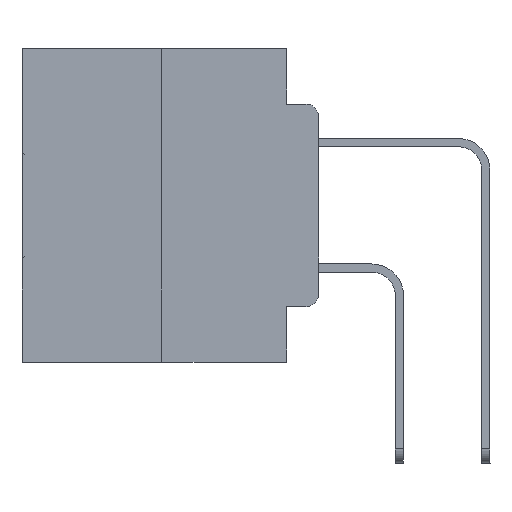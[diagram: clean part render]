
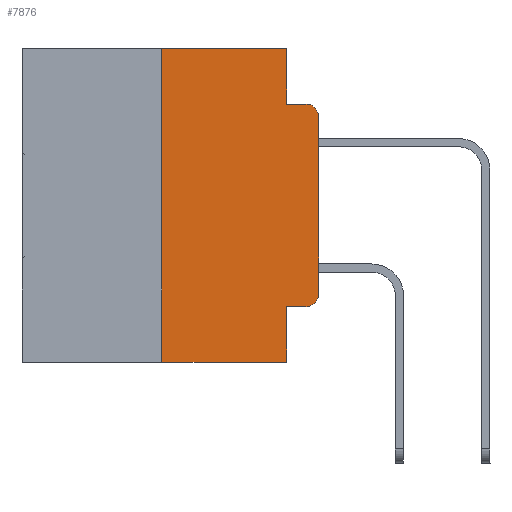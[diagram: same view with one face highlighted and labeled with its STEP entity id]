
A CAD part, left-side view. The second image highlights one B-rep face of the part: STEP entity #7876.
In plain terms, the highlighted planar face has unit normal (-1, 0, 0).
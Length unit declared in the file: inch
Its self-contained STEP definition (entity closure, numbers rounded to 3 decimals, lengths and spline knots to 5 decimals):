
#270 = VERTEX_POINT ( 'NONE', #4595 ) ;
#1238 = CARTESIAN_POINT ( 'NONE',  ( 0., 0.02, -0.3915 ) ) ;
#1372 = EDGE_CURVE ( 'NONE', #30174, #270, #13356, .T. ) ;
#1928 = VERTEX_POINT ( 'NONE', #25315 ) ;
#2842 = CARTESIAN_POINT ( 'NONE',  ( 0., 0.473, 0. ) ) ;
#2890 = VERTEX_POINT ( 'NONE', #15559 ) ;
#2945 = PLANE ( 'NONE',  #19170 ) ;
#3077 = EDGE_CURVE ( 'NONE', #2890, #270, #5493, .T. ) ;
#3279 = DIRECTION ( 'NONE',  ( 0., 0., 1. ) ) ;
#3811 = DIRECTION ( 'NONE',  ( 0., 0., -1. ) ) ;
#4303 = DIRECTION ( 'NONE',  ( 0., 0., -1. ) ) ;
#4576 = ORIENTED_EDGE ( 'NONE', *, *, #26491, .F. ) ;
#4595 = CARTESIAN_POINT ( 'NONE',  ( 0., 0.02, -0.0885 ) ) ;
#4787 = EDGE_CURVE ( 'NONE', #20805, #2890, #20725, .T. ) ;
#4844 = EDGE_LOOP ( 'NONE', ( #20172, #8056, #9629, #22399, #29525, #4576, #11192, #5338, #24660, #26188 ) ) ;
#4935 = VECTOR ( 'NONE', #18849, 39.37008 ) ;
#5258 = VECTOR ( 'NONE', #24513, 39.37008 ) ;
#5312 = LINE ( 'NONE', #20573, #29499 ) ;
#5338 = ORIENTED_EDGE ( 'NONE', *, *, #21654, .F. ) ;
#5465 = DIRECTION ( 'NONE',  ( 1., 0., 0. ) ) ;
#5493 = CIRCLE ( 'NONE', #10427, 0.02 ) ;
#5807 = CARTESIAN_POINT ( 'NONE',  ( 0., 0., 0. ) ) ;
#6363 = LINE ( 'NONE', #30226, #18552 ) ;
#6701 = CARTESIAN_POINT ( 'NONE',  ( 0., 0.25, -0.5 ) ) ;
#6771 = VECTOR ( 'NONE', #21631, 39.37008 ) ;
#6931 = DIRECTION ( 'NONE',  ( -1., 0., 0. ) ) ;
#7005 = CARTESIAN_POINT ( 'NONE',  ( 0., 0.02, -0.1085 ) ) ;
#7876 = ADVANCED_FACE ( 'NONE', ( #16884 ), #2945, .F. ) ;
#8056 = ORIENTED_EDGE ( 'NONE', *, *, #3077, .T. ) ;
#9015 = LINE ( 'NONE', #31048, #14792 ) ;
#9629 = ORIENTED_EDGE ( 'NONE', *, *, #1372, .F. ) ;
#10427 = AXIS2_PLACEMENT_3D ( 'NONE', #7005, #6931, #4303 ) ;
#11192 = ORIENTED_EDGE ( 'NONE', *, *, #26910, .T. ) ;
#11293 = CARTESIAN_POINT ( 'NONE',  ( 0., 0.051, -0.0885 ) ) ;
#11627 = CARTESIAN_POINT ( 'NONE',  ( 0., 0.25, 0. ) ) ;
#11630 = VERTEX_POINT ( 'NONE', #6701 ) ;
#12030 = CARTESIAN_POINT ( 'NONE',  ( 0., 0.051, 0. ) ) ;
#12297 = EDGE_CURVE ( 'NONE', #1928, #14678, #9015, .T. ) ;
#12622 = CARTESIAN_POINT ( 'NONE',  ( 0., 0.051, 0. ) ) ;
#13356 = LINE ( 'NONE', #11293, #6771 ) ;
#14461 = DIRECTION ( 'NONE',  ( 0., -1., 0. ) ) ;
#14678 = VERTEX_POINT ( 'NONE', #12030 ) ;
#14792 = VECTOR ( 'NONE', #14461, 39.37008 ) ;
#15109 = VERTEX_POINT ( 'NONE', #23163 ) ;
#15559 = CARTESIAN_POINT ( 'NONE',  ( 0., 0., -0.1085 ) ) ;
#16431 = LINE ( 'NONE', #17887, #28388 ) ;
#16884 = FACE_OUTER_BOUND ( 'NONE', #4844, .T. ) ;
#17194 = VERTEX_POINT ( 'NONE', #22791 ) ;
#17519 = LINE ( 'NONE', #12622, #5258 ) ;
#17887 = CARTESIAN_POINT ( 'NONE',  ( 0., 0.473, -0.5 ) ) ;
#17980 = AXIS2_PLACEMENT_3D ( 'NONE', #1238, #18458, #3811 ) ;
#18277 = DIRECTION ( 'NONE',  ( 0., -1., 0. ) ) ;
#18353 = DIRECTION ( 'NONE',  ( 0., 0., -1. ) ) ;
#18458 = DIRECTION ( 'NONE',  ( -1., 0., 0. ) ) ;
#18466 = EDGE_CURVE ( 'NONE', #17194, #20805, #24355, .T. ) ;
#18552 = VECTOR ( 'NONE', #18353, 39.37008 ) ;
#18849 = DIRECTION ( 'NONE',  ( 0., 0., 1. ) ) ;
#19170 = AXIS2_PLACEMENT_3D ( 'NONE', #2842, #5465, #22418 ) ;
#20070 = EDGE_CURVE ( 'NONE', #15109, #17194, #5312, .T. ) ;
#20172 = ORIENTED_EDGE ( 'NONE', *, *, #4787, .T. ) ;
#20573 = CARTESIAN_POINT ( 'NONE',  ( 0., 0.051, -0.4115 ) ) ;
#20725 = LINE ( 'NONE', #5807, #25587 ) ;
#20805 = VERTEX_POINT ( 'NONE', #25870 ) ;
#21631 = DIRECTION ( 'NONE',  ( 0., -1., 0. ) ) ;
#21654 = EDGE_CURVE ( 'NONE', #15109, #24845, #17519, .T. ) ;
#22399 = ORIENTED_EDGE ( 'NONE', *, *, #28108, .F. ) ;
#22418 = DIRECTION ( 'NONE',  ( 0., 0., -1. ) ) ;
#22749 = LINE ( 'NONE', #11627, #4935 ) ;
#22791 = CARTESIAN_POINT ( 'NONE',  ( 0., 0.02, -0.4115 ) ) ;
#23163 = CARTESIAN_POINT ( 'NONE',  ( 0., 0.051, -0.4115 ) ) ;
#24344 = CARTESIAN_POINT ( 'NONE',  ( 0., 0.051, -0.5 ) ) ;
#24355 = CIRCLE ( 'NONE', #17980, 0.02 ) ;
#24513 = DIRECTION ( 'NONE',  ( 0., 0., -1. ) ) ;
#24660 = ORIENTED_EDGE ( 'NONE', *, *, #20070, .T. ) ;
#24845 = VERTEX_POINT ( 'NONE', #24344 ) ;
#25065 = DIRECTION ( 'NONE',  ( 0., -1., 0. ) ) ;
#25315 = CARTESIAN_POINT ( 'NONE',  ( 0., 0.25, 0. ) ) ;
#25587 = VECTOR ( 'NONE', #3279, 39.37008 ) ;
#25870 = CARTESIAN_POINT ( 'NONE',  ( 0., 0., -0.3915 ) ) ;
#26188 = ORIENTED_EDGE ( 'NONE', *, *, #18466, .T. ) ;
#26491 = EDGE_CURVE ( 'NONE', #11630, #1928, #22749, .T. ) ;
#26910 = EDGE_CURVE ( 'NONE', #11630, #24845, #16431, .T. ) ;
#28108 = EDGE_CURVE ( 'NONE', #14678, #30174, #6363, .T. ) ;
#28388 = VECTOR ( 'NONE', #25065, 39.37008 ) ;
#28704 = CARTESIAN_POINT ( 'NONE',  ( 0., 0.051, -0.0885 ) ) ;
#29499 = VECTOR ( 'NONE', #18277, 39.37008 ) ;
#29525 = ORIENTED_EDGE ( 'NONE', *, *, #12297, .F. ) ;
#30174 = VERTEX_POINT ( 'NONE', #28704 ) ;
#30226 = CARTESIAN_POINT ( 'NONE',  ( 0., 0.051, 0. ) ) ;
#31048 = CARTESIAN_POINT ( 'NONE',  ( 0., 0.473, 0. ) ) ;
